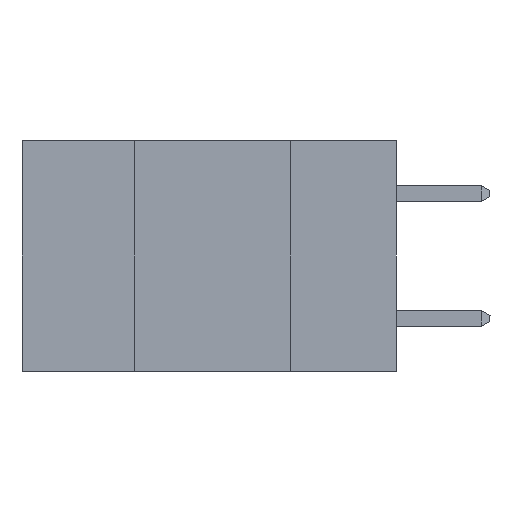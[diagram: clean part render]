
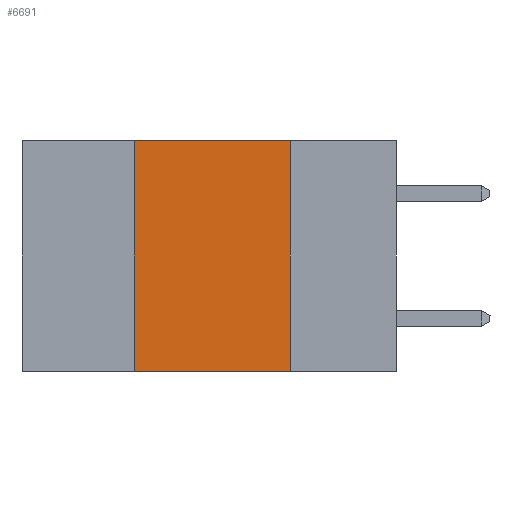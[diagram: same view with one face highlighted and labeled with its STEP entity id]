
A CAD part, left-side view. The second image highlights one B-rep face of the part: STEP entity #6691.
In plain terms, the highlighted planar face has unit normal (-1, 0, 0).
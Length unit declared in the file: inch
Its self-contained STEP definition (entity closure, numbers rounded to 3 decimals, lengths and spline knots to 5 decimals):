
#43 = AXIS2_PLACEMENT_3D ( 'NONE', #4330, #22865, #13778 ) ;
#179 = DIRECTION ( 'NONE',  ( 0., 0., 1. ) ) ;
#347 = VERTEX_POINT ( 'NONE', #16885 ) ;
#1514 = LINE ( 'NONE', #15117, #12396 ) ;
#1595 = VECTOR ( 'NONE', #6393, 39.37008 ) ;
#2471 = ORIENTED_EDGE ( 'NONE', *, *, #22430, .F. ) ;
#3011 = ORIENTED_EDGE ( 'NONE', *, *, #9734, .F. ) ;
#4330 = CARTESIAN_POINT ( 'NONE',  ( 0., 0.6, 0. ) ) ;
#6349 = CARTESIAN_POINT ( 'NONE',  ( 0., 0.42, -0.37 ) ) ;
#6393 = DIRECTION ( 'NONE',  ( 0., -1., 0. ) ) ;
#6691 = ADVANCED_FACE ( 'NONE', ( #22660 ), #10091, .F. ) ;
#7071 = DIRECTION ( 'NONE',  ( 0., -1., 0. ) ) ;
#7408 = VERTEX_POINT ( 'NONE', #15766 ) ;
#7630 = LINE ( 'NONE', #8412, #1595 ) ;
#8412 = CARTESIAN_POINT ( 'NONE',  ( 0., 0.6, -0.37 ) ) ;
#9734 = EDGE_CURVE ( 'NONE', #10277, #347, #1514, .T. ) ;
#10091 = PLANE ( 'NONE',  #43 ) ;
#10277 = VERTEX_POINT ( 'NONE', #6349 ) ;
#11422 = ORIENTED_EDGE ( 'NONE', *, *, #14151, .T. ) ;
#12396 = VECTOR ( 'NONE', #179, 39.37008 ) ;
#13087 = ORIENTED_EDGE ( 'NONE', *, *, #13153, .F. ) ;
#13153 = EDGE_CURVE ( 'NONE', #347, #7408, #18537, .T. ) ;
#13253 = VECTOR ( 'NONE', #18055, 39.37008 ) ;
#13398 = VECTOR ( 'NONE', #7071, 39.37008 ) ;
#13778 = DIRECTION ( 'NONE',  ( 0., 0., -1. ) ) ;
#13813 = LINE ( 'NONE', #16531, #13253 ) ;
#14151 = EDGE_CURVE ( 'NONE', #10277, #16888, #7630, .T. ) ;
#14738 = EDGE_LOOP ( 'NONE', ( #2471, #13087, #3011, #11422 ) ) ;
#15117 = CARTESIAN_POINT ( 'NONE',  ( 0., 0.42, 0. ) ) ;
#15766 = CARTESIAN_POINT ( 'NONE',  ( 0., 0.17, 0. ) ) ;
#16531 = CARTESIAN_POINT ( 'NONE',  ( 0., 0.17, 0. ) ) ;
#16885 = CARTESIAN_POINT ( 'NONE',  ( 0., 0.42, 0. ) ) ;
#16888 = VERTEX_POINT ( 'NONE', #22960 ) ;
#18001 = CARTESIAN_POINT ( 'NONE',  ( 0., 0.6, 0. ) ) ;
#18055 = DIRECTION ( 'NONE',  ( 0., 0., -1. ) ) ;
#18537 = LINE ( 'NONE', #18001, #13398 ) ;
#22430 = EDGE_CURVE ( 'NONE', #7408, #16888, #13813, .T. ) ;
#22660 = FACE_OUTER_BOUND ( 'NONE', #14738, .T. ) ;
#22865 = DIRECTION ( 'NONE',  ( 1., 0., 0. ) ) ;
#22960 = CARTESIAN_POINT ( 'NONE',  ( 0., 0.17, -0.37 ) ) ;
